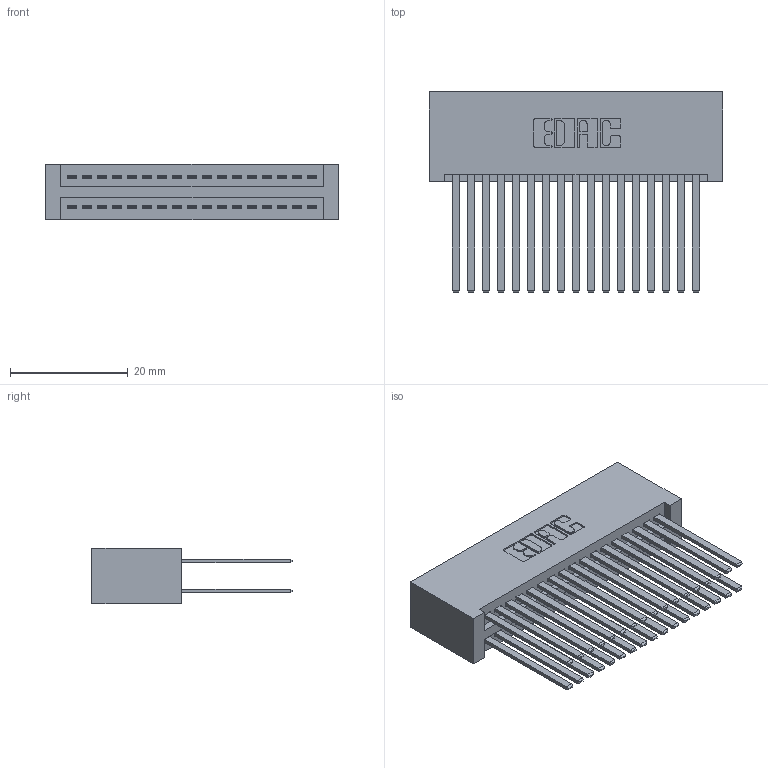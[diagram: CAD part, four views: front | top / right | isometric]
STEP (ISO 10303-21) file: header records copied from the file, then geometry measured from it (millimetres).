
FILE_DESCRIPTION (( 'STEP AP203' ), '1' );
FILE_NAME ('395-034-544-201.STEP', '2018-11-13T08:40:48', ( '' ), ( '' ), 'SwSTEP 2.0', 'SolidWorks 2016', '' );
FILE_SCHEMA (( 'CONFIG_CONTROL_DESIGN' ));
Length unit declared in the file: inch
Products named in the file (3): 395-034-544-201; 345 Part_No Mounting Lugs; 345-292-001_345-293-144
Assembly tree (35 placements, depth 2):
  395-034-544-201
    345 Part_No Mounting Lugs
    345-292-001_345-293-144  x34
Bounding box: 49.78 x 33.96 x 9.4 mm (x, y, z)
Volume: 5696.5 mm3; surface area: 9636.4 mm2
Topology: 35 solids, 35 shells, 1614 faces, 4771 edges, 3134 vertices
Faces by surface type: plane 1062, cylinder 552
Entity records: 16243 total; most frequent: CARTESIAN_POINT 2744, ORIENTED_EDGE 2678, DIRECTION 2443, EDGE_CURVE 1339, VECTOR 1151, LINE 1151, VERTEX_POINT 890, AXIS2_PLACEMENT_3D 646
